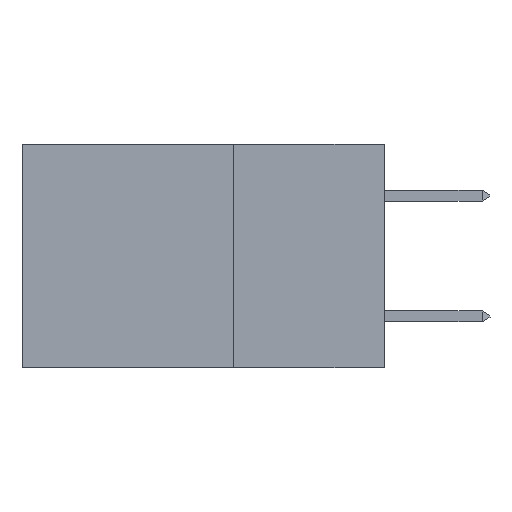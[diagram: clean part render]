
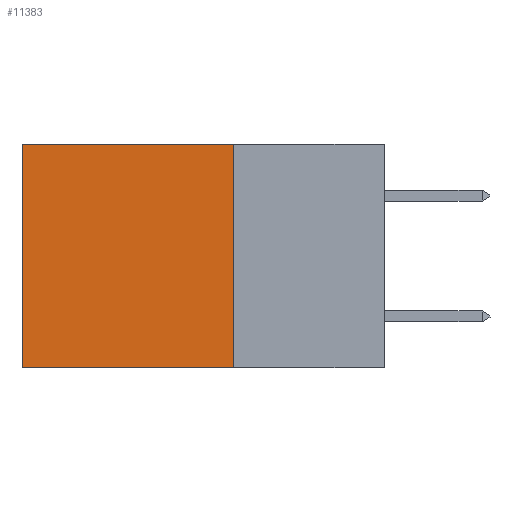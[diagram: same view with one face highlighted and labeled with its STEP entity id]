
A CAD part, left-side view. The second image highlights one B-rep face of the part: STEP entity #11383.
In plain terms, the highlighted planar face has unit normal (-1, 0, 0).
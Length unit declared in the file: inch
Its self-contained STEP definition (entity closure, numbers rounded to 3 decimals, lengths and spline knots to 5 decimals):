
#427 = DIRECTION ( 'NONE',  ( 0., 0., -1. ) ) ;
#803 = CARTESIAN_POINT ( 'NONE',  ( 0.2875, 0.25, -0.37 ) ) ;
#1880 = EDGE_CURVE ( 'NONE', #12201, #17484, #23658, .T. ) ;
#2276 = CARTESIAN_POINT ( 'NONE',  ( 0.2875, 0.25, 0. ) ) ;
#2984 = VECTOR ( 'NONE', #17802, 39.37008 ) ;
#3317 = LINE ( 'NONE', #16186, #12964 ) ;
#4132 = LINE ( 'NONE', #803, #8637 ) ;
#4639 = CARTESIAN_POINT ( 'NONE',  ( 0.2875, 0.6, 0. ) ) ;
#7018 = CARTESIAN_POINT ( 'NONE',  ( 0.2875, 0.6, 0. ) ) ;
#7928 = VERTEX_POINT ( 'NONE', #10460 ) ;
#8130 = CARTESIAN_POINT ( 'NONE',  ( 0.2875, 0.25, 0. ) ) ;
#8504 = EDGE_CURVE ( 'NONE', #21311, #7928, #4132, .T. ) ;
#8575 = DIRECTION ( 'NONE',  ( 0., 1., 0. ) ) ;
#8637 = VECTOR ( 'NONE', #8575, 39.37008 ) ;
#8796 = FACE_OUTER_BOUND ( 'NONE', #9421, .T. ) ;
#9421 = EDGE_LOOP ( 'NONE', ( #22916, #24306, #17531, #18348 ) ) ;
#10074 = PLANE ( 'NONE',  #21649 ) ;
#10081 = VECTOR ( 'NONE', #15666, 39.37008 ) ;
#10459 = CARTESIAN_POINT ( 'NONE',  ( 0.2875, 0.25, 0. ) ) ;
#10460 = CARTESIAN_POINT ( 'NONE',  ( 0.2875, 0.6, -0.37 ) ) ;
#11383 = ADVANCED_FACE ( 'NONE', ( #8796 ), #10074, .F. ) ;
#12037 = DIRECTION ( 'NONE',  ( 1., 0., 0. ) ) ;
#12201 = VERTEX_POINT ( 'NONE', #10459 ) ;
#12964 = VECTOR ( 'NONE', #17950, 39.37008 ) ;
#15666 = DIRECTION ( 'NONE',  ( 0., 1., 0. ) ) ;
#16186 = CARTESIAN_POINT ( 'NONE',  ( 0.2875, 0.25, 0. ) ) ;
#17484 = VERTEX_POINT ( 'NONE', #7018 ) ;
#17531 = ORIENTED_EDGE ( 'NONE', *, *, #21158, .F. ) ;
#17802 = DIRECTION ( 'NONE',  ( 0., 0., -1. ) ) ;
#17950 = DIRECTION ( 'NONE',  ( 0., 0., -1. ) ) ;
#18348 = ORIENTED_EDGE ( 'NONE', *, *, #1880, .T. ) ;
#19216 = EDGE_CURVE ( 'NONE', #17484, #7928, #22335, .T. ) ;
#20078 = CARTESIAN_POINT ( 'NONE',  ( 0.2875, 0.25, -0.37 ) ) ;
#21158 = EDGE_CURVE ( 'NONE', #12201, #21311, #3317, .T. ) ;
#21311 = VERTEX_POINT ( 'NONE', #20078 ) ;
#21649 = AXIS2_PLACEMENT_3D ( 'NONE', #8130, #12037, #427 ) ;
#22335 = LINE ( 'NONE', #4639, #2984 ) ;
#22916 = ORIENTED_EDGE ( 'NONE', *, *, #19216, .T. ) ;
#23658 = LINE ( 'NONE', #2276, #10081 ) ;
#24306 = ORIENTED_EDGE ( 'NONE', *, *, #8504, .F. ) ;
